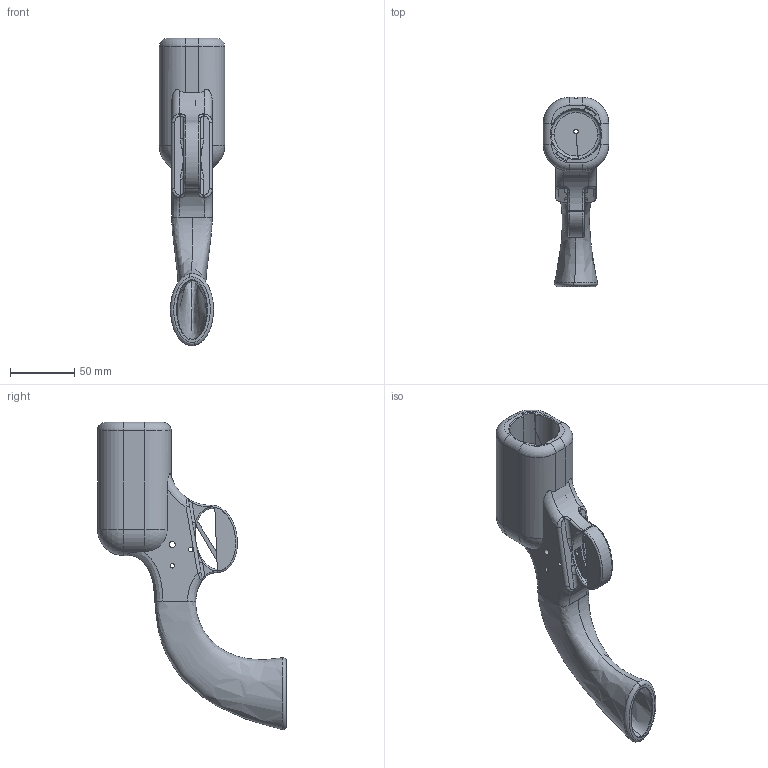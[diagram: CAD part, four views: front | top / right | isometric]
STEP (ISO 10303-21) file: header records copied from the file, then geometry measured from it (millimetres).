
FILE_DESCRIPTION (( 'STEP AP214' ), '1' );
FILE_NAME ('receiverhandgun.STEP', '2013-10-27T06:42:12', ( 'Matt' ), ( '' ), 'SwSTEP 2.0', 'SolidWorks 2013', '' );
FILE_SCHEMA (( 'AUTOMOTIVE_DESIGN' ));
Length unit declared in the file: inch
Products named in the file (1): receiverhandgun
Bounding box: 50.8 x 146.74 x 238.73 mm (x, y, z)
Volume: 251158.6 mm3; surface area: 73444.4 mm2
Topology: 2 solids, 2 shells, 216 faces, 569 edges, 356 vertices
Faces by surface type: cylinder 72, plane 66, bspline 53, cone 11, torus 10, sphere 4
Entity records: 15033 total; most frequent: CARTESIAN_POINT 10053, ORIENTED_EDGE 1134, DIRECTION 892, EDGE_CURVE 567, VERTEX_POINT 356, AXIS2_PLACEMENT_3D 344, EDGE_LOOP 237, ADVANCED_FACE 216
